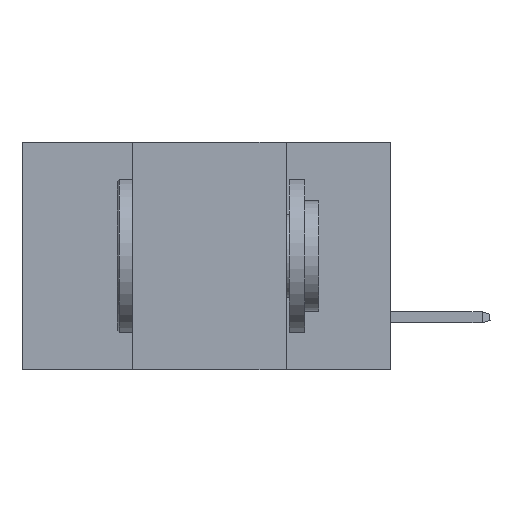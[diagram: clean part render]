
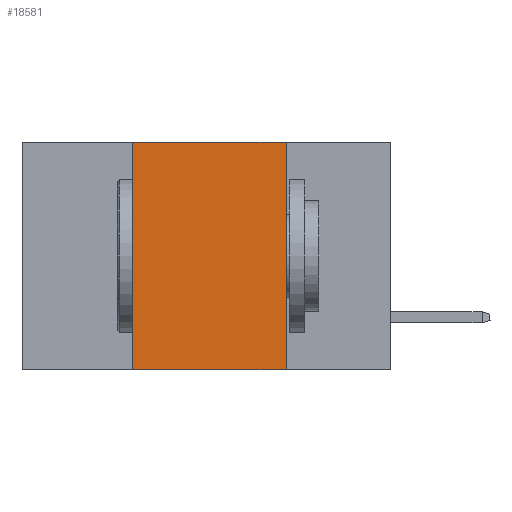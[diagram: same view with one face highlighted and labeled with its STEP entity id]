
A CAD part, left-side view. The second image highlights one B-rep face of the part: STEP entity #18581.
In plain terms, the highlighted planar face has unit normal (-1, 0, 0).
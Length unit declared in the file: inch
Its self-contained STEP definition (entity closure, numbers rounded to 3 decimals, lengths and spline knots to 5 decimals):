
#390 = EDGE_LOOP ( 'NONE', ( #18718, #36655, #6802, #39502 ) ) ;
#1053 = VERTEX_POINT ( 'NONE', #37542 ) ;
#3286 = VERTEX_POINT ( 'NONE', #10090 ) ;
#3577 = VERTEX_POINT ( 'NONE', #15927 ) ;
#4669 = LINE ( 'NONE', #33077, #45260 ) ;
#5782 = DIRECTION ( 'NONE',  ( 0., -1., 0. ) ) ;
#6014 = PLANE ( 'NONE',  #37084 ) ;
#6802 = ORIENTED_EDGE ( 'NONE', *, *, #25102, .F. ) ;
#7971 = LINE ( 'NONE', #16655, #33314 ) ;
#10090 = CARTESIAN_POINT ( 'NONE',  ( 0., 0.17, -0.37 ) ) ;
#13573 = DIRECTION ( 'NONE',  ( 1., 0., 0. ) ) ;
#14977 = LINE ( 'NONE', #27241, #42020 ) ;
#15356 = EDGE_CURVE ( 'NONE', #3577, #1053, #14977, .T. ) ;
#15927 = CARTESIAN_POINT ( 'NONE',  ( 0., 0.42, 0. ) ) ;
#16655 = CARTESIAN_POINT ( 'NONE',  ( 0., 0.6, -0.37 ) ) ;
#17663 = CARTESIAN_POINT ( 'NONE',  ( 0., 0.6, 0. ) ) ;
#18581 = ADVANCED_FACE ( 'NONE', ( #29959 ), #6014, .F. ) ;
#18718 = ORIENTED_EDGE ( 'NONE', *, *, #41000, .F. ) ;
#23395 = LINE ( 'NONE', #24617, #23935 ) ;
#23935 = VECTOR ( 'NONE', #31211, 39.37008 ) ;
#24617 = CARTESIAN_POINT ( 'NONE',  ( 0., 0.42, 0. ) ) ;
#25102 = EDGE_CURVE ( 'NONE', #39587, #3577, #23395, .T. ) ;
#27241 = CARTESIAN_POINT ( 'NONE',  ( 0., 0.6, 0. ) ) ;
#29959 = FACE_OUTER_BOUND ( 'NONE', #390, .T. ) ;
#30593 = DIRECTION ( 'NONE',  ( 0., -1., 0. ) ) ;
#31211 = DIRECTION ( 'NONE',  ( 0., 0., 1. ) ) ;
#31635 = DIRECTION ( 'NONE',  ( 0., 0., -1. ) ) ;
#33077 = CARTESIAN_POINT ( 'NONE',  ( 0., 0.17, 0. ) ) ;
#33314 = VECTOR ( 'NONE', #5782, 39.37008 ) ;
#35133 = EDGE_CURVE ( 'NONE', #39587, #3286, #7971, .T. ) ;
#36655 = ORIENTED_EDGE ( 'NONE', *, *, #15356, .F. ) ;
#36856 = DIRECTION ( 'NONE',  ( 0., 0., -1. ) ) ;
#37084 = AXIS2_PLACEMENT_3D ( 'NONE', #17663, #13573, #31635 ) ;
#37542 = CARTESIAN_POINT ( 'NONE',  ( 0., 0.17, 0. ) ) ;
#39502 = ORIENTED_EDGE ( 'NONE', *, *, #35133, .T. ) ;
#39587 = VERTEX_POINT ( 'NONE', #44780 ) ;
#41000 = EDGE_CURVE ( 'NONE', #1053, #3286, #4669, .T. ) ;
#42020 = VECTOR ( 'NONE', #30593, 39.37008 ) ;
#44780 = CARTESIAN_POINT ( 'NONE',  ( 0., 0.42, -0.37 ) ) ;
#45260 = VECTOR ( 'NONE', #36856, 39.37008 ) ;
